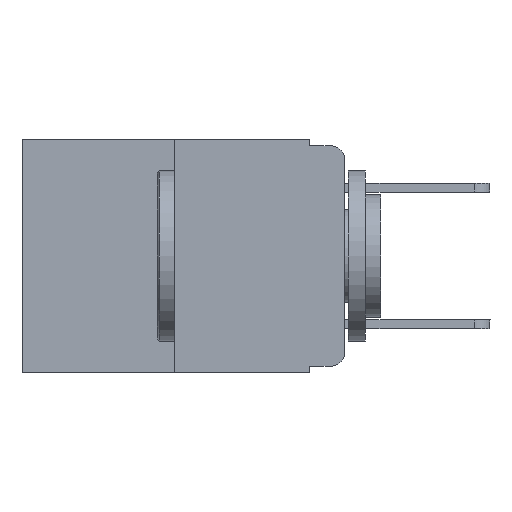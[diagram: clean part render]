
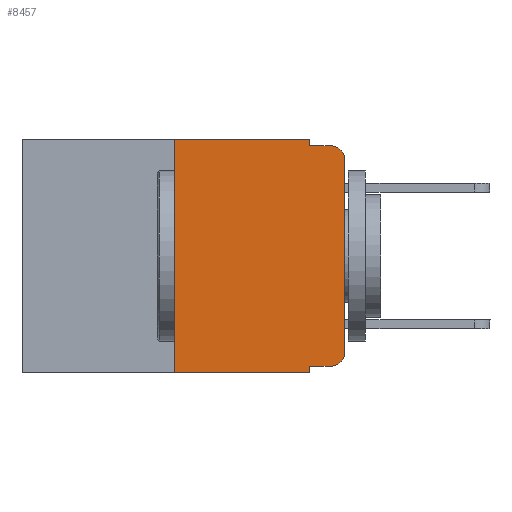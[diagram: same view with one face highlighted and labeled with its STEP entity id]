
A CAD part, left-side view. The second image highlights one B-rep face of the part: STEP entity #8457.
In plain terms, the highlighted planar face has unit normal (-1, 0, 0).
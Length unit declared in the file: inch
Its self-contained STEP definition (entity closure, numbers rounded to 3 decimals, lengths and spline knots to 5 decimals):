
#166 = ORIENTED_EDGE ( 'NONE', *, *, #11187, .F. ) ;
#330 = VERTEX_POINT ( 'NONE', #1908 ) ;
#407 = EDGE_CURVE ( 'NONE', #2988, #8939, #6179, .T. ) ;
#508 = VERTEX_POINT ( 'NONE', #1092 ) ;
#560 = CARTESIAN_POINT ( 'NONE',  ( 0., 0.25, 0. ) ) ;
#968 = LINE ( 'NONE', #7512, #3361 ) ;
#1092 = CARTESIAN_POINT ( 'NONE',  ( 0., 0., -0.03 ) ) ;
#1335 = CIRCLE ( 'NONE', #5883, 0.02 ) ;
#1448 = DIRECTION ( 'NONE',  ( 0., -1., 0. ) ) ;
#1481 = EDGE_CURVE ( 'NONE', #8191, #2227, #11156, .T. ) ;
#1680 = DIRECTION ( 'NONE',  ( -1., 0., 0. ) ) ;
#1793 = DIRECTION ( 'NONE',  ( 0., 0., -1. ) ) ;
#1804 = AXIS2_PLACEMENT_3D ( 'NONE', #2609, #1680, #6851 ) ;
#1858 = EDGE_CURVE ( 'NONE', #8191, #6906, #6900, .T. ) ;
#1908 = CARTESIAN_POINT ( 'NONE',  ( 0., 0.25, -0.343 ) ) ;
#1963 = CIRCLE ( 'NONE', #1804, 0.02 ) ;
#2093 = CARTESIAN_POINT ( 'NONE',  ( 0., 0.02, -0.01 ) ) ;
#2170 = DIRECTION ( 'NONE',  ( 0., 0., 1. ) ) ;
#2227 = VERTEX_POINT ( 'NONE', #9559 ) ;
#2475 = VECTOR ( 'NONE', #8379, 39.37008 ) ;
#2609 = CARTESIAN_POINT ( 'NONE',  ( 0., 0.02, -0.313 ) ) ;
#2672 = ORIENTED_EDGE ( 'NONE', *, *, #8754, .F. ) ;
#2780 = LINE ( 'NONE', #3062, #12271 ) ;
#2988 = VERTEX_POINT ( 'NONE', #10386 ) ;
#3062 = CARTESIAN_POINT ( 'NONE',  ( 0., 0.051, 0. ) ) ;
#3099 = EDGE_CURVE ( 'NONE', #8060, #11295, #968, .T. ) ;
#3135 = CARTESIAN_POINT ( 'NONE',  ( 0., 0.25, 0. ) ) ;
#3210 = CARTESIAN_POINT ( 'NONE',  ( 0., 0., -0.313 ) ) ;
#3361 = VECTOR ( 'NONE', #9580, 39.37008 ) ;
#3387 = CARTESIAN_POINT ( 'NONE',  ( 0., 0.051, -0.333 ) ) ;
#3534 = DIRECTION ( 'NONE',  ( 0., 0., -1. ) ) ;
#3812 = DIRECTION ( 'NONE',  ( 1., 0., 0. ) ) ;
#3833 = ORIENTED_EDGE ( 'NONE', *, *, #6211, .T. ) ;
#3948 = LINE ( 'NONE', #12268, #9472 ) ;
#4195 = ORIENTED_EDGE ( 'NONE', *, *, #407, .F. ) ;
#4374 = CARTESIAN_POINT ( 'NONE',  ( 0., 0.02, -0.03 ) ) ;
#4590 = AXIS2_PLACEMENT_3D ( 'NONE', #7895, #3812, #1793 ) ;
#4889 = LINE ( 'NONE', #10579, #8362 ) ;
#5206 = DIRECTION ( 'NONE',  ( 0., 0., -1. ) ) ;
#5809 = VERTEX_POINT ( 'NONE', #3210 ) ;
#5883 = AXIS2_PLACEMENT_3D ( 'NONE', #4374, #9598, #3534 ) ;
#5969 = VECTOR ( 'NONE', #11579, 39.37008 ) ;
#6179 = LINE ( 'NONE', #11120, #2475 ) ;
#6211 = EDGE_CURVE ( 'NONE', #5809, #508, #3948, .T. ) ;
#6242 = ORIENTED_EDGE ( 'NONE', *, *, #1858, .F. ) ;
#6495 = EDGE_CURVE ( 'NONE', #330, #6906, #4889, .T. ) ;
#6498 = ORIENTED_EDGE ( 'NONE', *, *, #1481, .T. ) ;
#6657 = LINE ( 'NONE', #560, #10105 ) ;
#6746 = DIRECTION ( 'NONE',  ( 0., 0., 1. ) ) ;
#6851 = DIRECTION ( 'NONE',  ( 0., 0., -1. ) ) ;
#6900 = LINE ( 'NONE', #10647, #7522 ) ;
#6906 = VERTEX_POINT ( 'NONE', #8108 ) ;
#7017 = ORIENTED_EDGE ( 'NONE', *, *, #6495, .T. ) ;
#7063 = EDGE_CURVE ( 'NONE', #508, #8939, #1335, .T. ) ;
#7220 = ORIENTED_EDGE ( 'NONE', *, *, #11530, .T. ) ;
#7512 = CARTESIAN_POINT ( 'NONE',  ( 0., 0.473, 0. ) ) ;
#7522 = VECTOR ( 'NONE', #11734, 39.37008 ) ;
#7618 = PLANE ( 'NONE',  #4590 ) ;
#7895 = CARTESIAN_POINT ( 'NONE',  ( 0., 0.473, 0. ) ) ;
#8060 = VERTEX_POINT ( 'NONE', #3135 ) ;
#8108 = CARTESIAN_POINT ( 'NONE',  ( 0., 0.051, -0.343 ) ) ;
#8191 = VERTEX_POINT ( 'NONE', #9418 ) ;
#8362 = VECTOR ( 'NONE', #1448, 39.37008 ) ;
#8379 = DIRECTION ( 'NONE',  ( 0., -1., 0. ) ) ;
#8457 = ADVANCED_FACE ( 'NONE', ( #8475 ), #7618, .F. ) ;
#8475 = FACE_OUTER_BOUND ( 'NONE', #11717, .T. ) ;
#8754 = EDGE_CURVE ( 'NONE', #330, #8060, #6657, .T. ) ;
#8939 = VERTEX_POINT ( 'NONE', #2093 ) ;
#9348 = CARTESIAN_POINT ( 'NONE',  ( 0., 0.051, 0. ) ) ;
#9418 = CARTESIAN_POINT ( 'NONE',  ( 0., 0.051, -0.333 ) ) ;
#9472 = VECTOR ( 'NONE', #2170, 39.37008 ) ;
#9559 = CARTESIAN_POINT ( 'NONE',  ( 0., 0.02, -0.333 ) ) ;
#9580 = DIRECTION ( 'NONE',  ( 0., -1., 0. ) ) ;
#9598 = DIRECTION ( 'NONE',  ( -1., 0., 0. ) ) ;
#10011 = ORIENTED_EDGE ( 'NONE', *, *, #3099, .F. ) ;
#10105 = VECTOR ( 'NONE', #6746, 39.37008 ) ;
#10386 = CARTESIAN_POINT ( 'NONE',  ( 0., 0.051, -0.01 ) ) ;
#10579 = CARTESIAN_POINT ( 'NONE',  ( 0., 0.473, -0.343 ) ) ;
#10647 = CARTESIAN_POINT ( 'NONE',  ( 0., 0.051, 0. ) ) ;
#11120 = CARTESIAN_POINT ( 'NONE',  ( 0., 0.051, -0.01 ) ) ;
#11156 = LINE ( 'NONE', #3387, #5969 ) ;
#11187 = EDGE_CURVE ( 'NONE', #11295, #2988, #2780, .T. ) ;
#11295 = VERTEX_POINT ( 'NONE', #9348 ) ;
#11530 = EDGE_CURVE ( 'NONE', #2227, #5809, #1963, .T. ) ;
#11579 = DIRECTION ( 'NONE',  ( 0., -1., 0. ) ) ;
#11717 = EDGE_LOOP ( 'NONE', ( #3833, #11910, #4195, #166, #10011, #2672, #7017, #6242, #6498, #7220 ) ) ;
#11734 = DIRECTION ( 'NONE',  ( 0., 0., -1. ) ) ;
#11910 = ORIENTED_EDGE ( 'NONE', *, *, #7063, .T. ) ;
#12268 = CARTESIAN_POINT ( 'NONE',  ( 0., 0., 0. ) ) ;
#12271 = VECTOR ( 'NONE', #5206, 39.37008 ) ;
